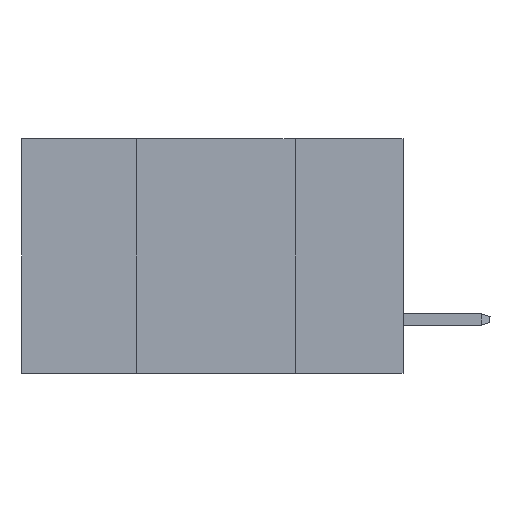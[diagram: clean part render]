
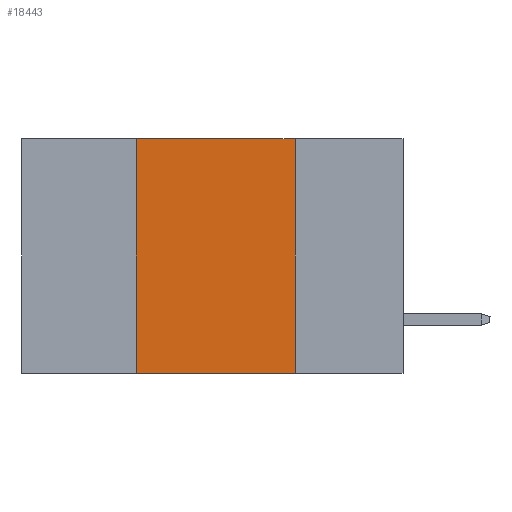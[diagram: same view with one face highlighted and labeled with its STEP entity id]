
A CAD part, left-side view. The second image highlights one B-rep face of the part: STEP entity #18443.
In plain terms, the highlighted planar face has unit normal (-1, 0, 0).
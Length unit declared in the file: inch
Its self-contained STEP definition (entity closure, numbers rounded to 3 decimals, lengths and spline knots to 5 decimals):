
#382 = EDGE_CURVE ( 'NONE', #22458, #19891, #21137, .T. ) ;
#1133 = AXIS2_PLACEMENT_3D ( 'NONE', #22384, #1641, #6891 ) ;
#1641 = DIRECTION ( 'NONE',  ( 1., 0., 0. ) ) ;
#2696 = ORIENTED_EDGE ( 'NONE', *, *, #6626, .F. ) ;
#2800 = ORIENTED_EDGE ( 'NONE', *, *, #9241, .F. ) ;
#2866 = VECTOR ( 'NONE', #10600, 39.37008 ) ;
#3010 = EDGE_LOOP ( 'NONE', ( #2696, #3541, #2800, #8344 ) ) ;
#3541 = ORIENTED_EDGE ( 'NONE', *, *, #16024, .F. ) ;
#3549 = LINE ( 'NONE', #5367, #2866 ) ;
#3799 = CARTESIAN_POINT ( 'NONE',  ( 0., 0.17, -0.37 ) ) ;
#5367 = CARTESIAN_POINT ( 'NONE',  ( 0., 0.42, 0. ) ) ;
#6283 = VECTOR ( 'NONE', #6771, 39.37008 ) ;
#6414 = CARTESIAN_POINT ( 'NONE',  ( 0., 0.42, -0.37 ) ) ;
#6626 = EDGE_CURVE ( 'NONE', #20846, #19891, #22498, .T. ) ;
#6659 = FACE_OUTER_BOUND ( 'NONE', #3010, .T. ) ;
#6771 = DIRECTION ( 'NONE',  ( 0., 0., -1. ) ) ;
#6891 = DIRECTION ( 'NONE',  ( 0., 0., -1. ) ) ;
#8344 = ORIENTED_EDGE ( 'NONE', *, *, #382, .T. ) ;
#9241 = EDGE_CURVE ( 'NONE', #22458, #13084, #3549, .T. ) ;
#10600 = DIRECTION ( 'NONE',  ( 0., 0., 1. ) ) ;
#12476 = CARTESIAN_POINT ( 'NONE',  ( 0., 0.6, -0.37 ) ) ;
#13084 = VERTEX_POINT ( 'NONE', #21415 ) ;
#14484 = CARTESIAN_POINT ( 'NONE',  ( 0., 0.6, 0. ) ) ;
#15246 = VECTOR ( 'NONE', #15968, 39.37008 ) ;
#15968 = DIRECTION ( 'NONE',  ( 0., -1., 0. ) ) ;
#16024 = EDGE_CURVE ( 'NONE', #13084, #20846, #17903, .T. ) ;
#17903 = LINE ( 'NONE', #14484, #15246 ) ;
#18443 = ADVANCED_FACE ( 'NONE', ( #6659 ), #19183, .F. ) ;
#19183 = PLANE ( 'NONE',  #1133 ) ;
#19891 = VERTEX_POINT ( 'NONE', #3799 ) ;
#20389 = DIRECTION ( 'NONE',  ( 0., -1., 0. ) ) ;
#20557 = CARTESIAN_POINT ( 'NONE',  ( 0., 0.17, 0. ) ) ;
#20667 = VECTOR ( 'NONE', #20389, 39.37008 ) ;
#20772 = CARTESIAN_POINT ( 'NONE',  ( 0., 0.17, 0. ) ) ;
#20846 = VERTEX_POINT ( 'NONE', #20557 ) ;
#21137 = LINE ( 'NONE', #12476, #20667 ) ;
#21415 = CARTESIAN_POINT ( 'NONE',  ( 0., 0.42, 0. ) ) ;
#22384 = CARTESIAN_POINT ( 'NONE',  ( 0., 0.6, 0. ) ) ;
#22458 = VERTEX_POINT ( 'NONE', #6414 ) ;
#22498 = LINE ( 'NONE', #20772, #6283 ) ;
